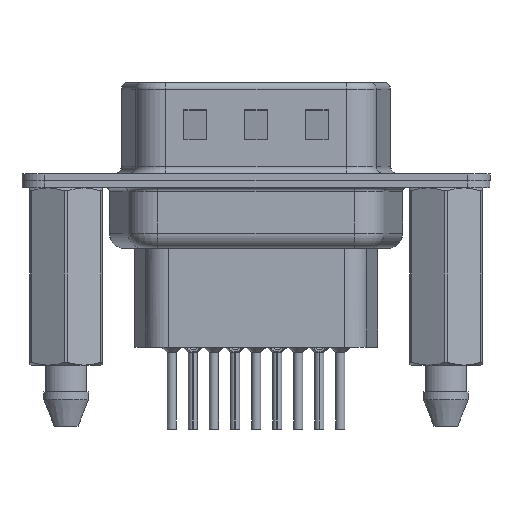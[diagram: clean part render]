
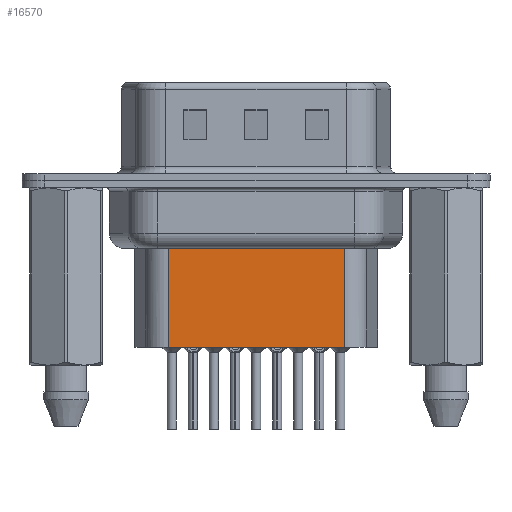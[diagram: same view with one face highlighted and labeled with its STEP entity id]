
A CAD part, front view. The second image highlights one B-rep face of the part: STEP entity #16570.
In plain terms, the highlighted planar face has unit normal (0, -1, 0).
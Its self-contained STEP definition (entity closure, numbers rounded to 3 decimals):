
#407 = DIRECTION ( 'NONE',  ( 0., 0., -1. ) ) ;
#649 = CARTESIAN_POINT ( 'NONE',  ( 18.294, -3.5, -10.95 ) ) ;
#1554 = CARTESIAN_POINT ( 'NONE',  ( 6.706, -3.5, -10.95 ) ) ;
#1569 = VERTEX_POINT ( 'NONE', #649 ) ;
#2345 = DIRECTION ( 'NONE',  ( 0., -1., 0. ) ) ;
#2452 = DIRECTION ( 'NONE',  ( 1., 0., 0. ) ) ;
#2593 = VECTOR ( 'NONE', #13494, 1000. ) ;
#4053 = VECTOR ( 'NONE', #6716, 1000. ) ;
#5492 = ORIENTED_EDGE ( 'NONE', *, *, #9102, .T. ) ;
#5587 = CARTESIAN_POINT ( 'NONE',  ( 6.706, -3.5, -4.097 ) ) ;
#6716 = DIRECTION ( 'NONE',  ( -1., 0., 0. ) ) ;
#8202 = VERTEX_POINT ( 'NONE', #20328 ) ;
#8319 = EDGE_CURVE ( 'NONE', #10462, #11876, #15416, .T. ) ;
#9102 = EDGE_CURVE ( 'NONE', #11876, #8202, #18822, .T. ) ;
#9337 = FACE_OUTER_BOUND ( 'NONE', #14185, .T. ) ;
#9687 = ORIENTED_EDGE ( 'NONE', *, *, #14252, .F. ) ;
#10352 = DIRECTION ( 'NONE',  ( -1., 0., 0. ) ) ;
#10462 = VERTEX_POINT ( 'NONE', #13846 ) ;
#10502 = CARTESIAN_POINT ( 'NONE',  ( 6.706, -3.5, -3.1 ) ) ;
#11876 = VERTEX_POINT ( 'NONE', #5587 ) ;
#12358 = PLANE ( 'NONE',  #16388 ) ;
#13494 = DIRECTION ( 'NONE',  ( 0., 0., -1. ) ) ;
#13665 = ORIENTED_EDGE ( 'NONE', *, *, #17973, .F. ) ;
#13846 = CARTESIAN_POINT ( 'NONE',  ( 18.294, -3.5, -4.097 ) ) ;
#14185 = EDGE_LOOP ( 'NONE', ( #9687, #19088, #5492, #13665 ) ) ;
#14252 = EDGE_CURVE ( 'NONE', #10462, #1569, #16626, .T. ) ;
#15102 = CARTESIAN_POINT ( 'NONE',  ( 18.294, -3.5, -3.1 ) ) ;
#15306 = CARTESIAN_POINT ( 'NONE',  ( 6.459, -3.5, -4.097 ) ) ;
#15416 = LINE ( 'NONE', #15306, #18749 ) ;
#15651 = VECTOR ( 'NONE', #407, 1000. ) ;
#16388 = AXIS2_PLACEMENT_3D ( 'NONE', #18729, #2345, #2452 ) ;
#16570 = ADVANCED_FACE ( 'NONE', ( #9337 ), #12358, .T. ) ;
#16626 = LINE ( 'NONE', #15102, #2593 ) ;
#17937 = LINE ( 'NONE', #1554, #4053 ) ;
#17973 = EDGE_CURVE ( 'NONE', #1569, #8202, #17937, .T. ) ;
#18729 = CARTESIAN_POINT ( 'NONE',  ( 6.706, -3.5, -3.1 ) ) ;
#18749 = VECTOR ( 'NONE', #10352, 1000. ) ;
#18822 = LINE ( 'NONE', #10502, #15651 ) ;
#19088 = ORIENTED_EDGE ( 'NONE', *, *, #8319, .T. ) ;
#20328 = CARTESIAN_POINT ( 'NONE',  ( 6.706, -3.5, -10.95 ) ) ;
